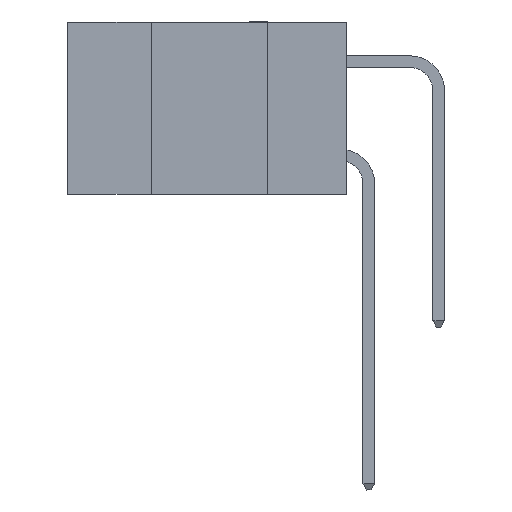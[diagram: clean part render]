
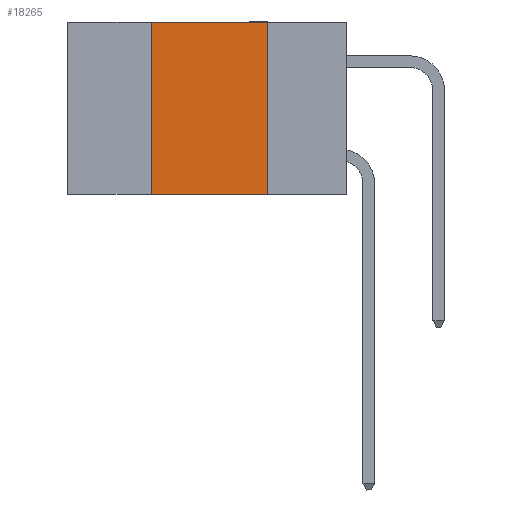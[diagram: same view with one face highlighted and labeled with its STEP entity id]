
A CAD part, left-side view. The second image highlights one B-rep face of the part: STEP entity #18265.
In plain terms, the highlighted planar face has unit normal (-1, 0, 0).
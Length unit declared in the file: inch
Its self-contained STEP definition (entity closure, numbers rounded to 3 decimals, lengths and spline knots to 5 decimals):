
#314 = VECTOR ( 'NONE', #3648, 39.37008 ) ;
#832 = ORIENTED_EDGE ( 'NONE', *, *, #6187, .F. ) ;
#1550 = EDGE_CURVE ( 'NONE', #8759, #10572, #2581, .T. ) ;
#2121 = VECTOR ( 'NONE', #6636, 39.37008 ) ;
#2176 = EDGE_CURVE ( 'NONE', #10572, #14979, #11157, .T. ) ;
#2220 = DIRECTION ( 'NONE',  ( 1., 0., 0. ) ) ;
#2334 = CARTESIAN_POINT ( 'NONE',  ( 0., 0.42, 0. ) ) ;
#2581 = LINE ( 'NONE', #2334, #2121 ) ;
#2868 = LINE ( 'NONE', #13776, #14625 ) ;
#3607 = ORIENTED_EDGE ( 'NONE', *, *, #2176, .F. ) ;
#3648 = DIRECTION ( 'NONE',  ( 0., 0., -1. ) ) ;
#4307 = VECTOR ( 'NONE', #12769, 39.37008 ) ;
#4553 = LINE ( 'NONE', #16270, #314 ) ;
#5078 = EDGE_LOOP ( 'NONE', ( #832, #3607, #13663, #14449 ) ) ;
#5292 = VERTEX_POINT ( 'NONE', #17112 ) ;
#5602 = CARTESIAN_POINT ( 'NONE',  ( 0., 0.42, 0. ) ) ;
#6187 = EDGE_CURVE ( 'NONE', #14979, #5292, #4553, .T. ) ;
#6636 = DIRECTION ( 'NONE',  ( 0., 0., 1. ) ) ;
#7880 = CARTESIAN_POINT ( 'NONE',  ( 0., 0.17, 0. ) ) ;
#8759 = VERTEX_POINT ( 'NONE', #10560 ) ;
#9840 = CARTESIAN_POINT ( 'NONE',  ( 0., 0.6, 0. ) ) ;
#10560 = CARTESIAN_POINT ( 'NONE',  ( 0., 0.42, -0.37 ) ) ;
#10572 = VERTEX_POINT ( 'NONE', #5602 ) ;
#10688 = CARTESIAN_POINT ( 'NONE',  ( 0., 0.6, 0. ) ) ;
#11157 = LINE ( 'NONE', #9840, #4307 ) ;
#12116 = DIRECTION ( 'NONE',  ( 0., 0., -1. ) ) ;
#12769 = DIRECTION ( 'NONE',  ( 0., -1., 0. ) ) ;
#13588 = DIRECTION ( 'NONE',  ( 0., -1., 0. ) ) ;
#13663 = ORIENTED_EDGE ( 'NONE', *, *, #1550, .F. ) ;
#13776 = CARTESIAN_POINT ( 'NONE',  ( 0., 0.6, -0.37 ) ) ;
#13894 = FACE_OUTER_BOUND ( 'NONE', #5078, .T. ) ;
#14449 = ORIENTED_EDGE ( 'NONE', *, *, #17366, .T. ) ;
#14625 = VECTOR ( 'NONE', #13588, 39.37008 ) ;
#14874 = AXIS2_PLACEMENT_3D ( 'NONE', #10688, #2220, #12116 ) ;
#14979 = VERTEX_POINT ( 'NONE', #7880 ) ;
#16270 = CARTESIAN_POINT ( 'NONE',  ( 0., 0.17, 0. ) ) ;
#17112 = CARTESIAN_POINT ( 'NONE',  ( 0., 0.17, -0.37 ) ) ;
#17366 = EDGE_CURVE ( 'NONE', #8759, #5292, #2868, .T. ) ;
#17697 = PLANE ( 'NONE',  #14874 ) ;
#18265 = ADVANCED_FACE ( 'NONE', ( #13894 ), #17697, .F. ) ;
